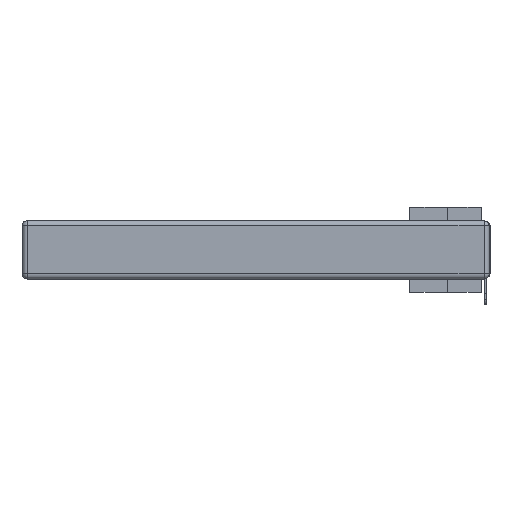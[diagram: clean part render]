
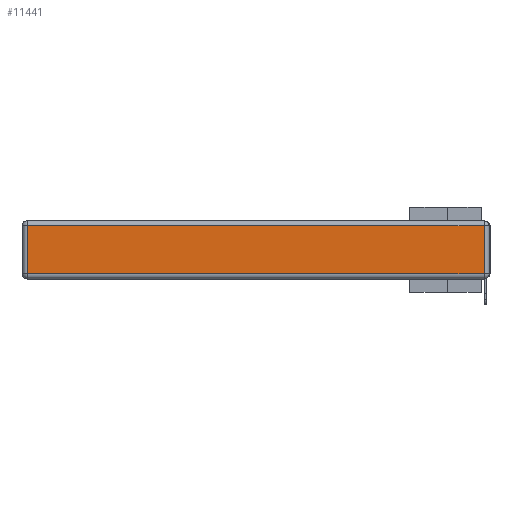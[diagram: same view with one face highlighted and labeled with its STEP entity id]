
A CAD part, left-side view. The second image highlights one B-rep face of the part: STEP entity #11441.
In plain terms, the highlighted planar face has unit normal (-1, 0, 0).
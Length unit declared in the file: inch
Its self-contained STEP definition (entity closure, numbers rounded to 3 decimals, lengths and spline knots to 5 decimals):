
#720 = LINE ( 'NONE', #28766, #16101 ) ;
#1318 = VERTEX_POINT ( 'NONE', #7488 ) ;
#3159 = ORIENTED_EDGE ( 'NONE', *, *, #16158, .T. ) ;
#4341 = DIRECTION ( 'NONE',  ( 0., 0., 1. ) ) ;
#7259 = VECTOR ( 'NONE', #16710, 39.37008 ) ;
#7416 = ORIENTED_EDGE ( 'NONE', *, *, #13104, .T. ) ;
#7488 = CARTESIAN_POINT ( 'NONE',  ( 0., 2.72, -0.313 ) ) ;
#7515 = CARTESIAN_POINT ( 'NONE',  ( 0., 0.03, -0.03 ) ) ;
#7822 = ORIENTED_EDGE ( 'NONE', *, *, #8214, .T. ) ;
#8214 = EDGE_CURVE ( 'NONE', #15928, #32894, #14979, .T. ) ;
#8232 = CARTESIAN_POINT ( 'NONE',  ( 0., 0., -0.343 ) ) ;
#10651 = PLANE ( 'NONE',  #28773 ) ;
#11441 = ADVANCED_FACE ( 'NONE', ( #14709 ), #10651, .T. ) ;
#11745 = CARTESIAN_POINT ( 'NONE',  ( 0., 2.72, -0.343 ) ) ;
#13104 = EDGE_CURVE ( 'NONE', #21676, #15928, #29478, .T. ) ;
#14709 = FACE_OUTER_BOUND ( 'NONE', #34022, .T. ) ;
#14979 = LINE ( 'NONE', #34029, #7259 ) ;
#15928 = VERTEX_POINT ( 'NONE', #7515 ) ;
#15938 = LINE ( 'NONE', #11745, #30003 ) ;
#16101 = VECTOR ( 'NONE', #34733, 39.37008 ) ;
#16158 = EDGE_CURVE ( 'NONE', #1318, #21676, #720, .T. ) ;
#16471 = ORIENTED_EDGE ( 'NONE', *, *, #27239, .T. ) ;
#16710 = DIRECTION ( 'NONE',  ( 0., 1., 0. ) ) ;
#20856 = VECTOR ( 'NONE', #4341, 39.37008 ) ;
#21676 = VERTEX_POINT ( 'NONE', #33018 ) ;
#21695 = CARTESIAN_POINT ( 'NONE',  ( 0., 0.03, -0.343 ) ) ;
#27239 = EDGE_CURVE ( 'NONE', #32894, #1318, #15938, .T. ) ;
#28766 = CARTESIAN_POINT ( 'NONE',  ( 0., 0., -0.313 ) ) ;
#28773 = AXIS2_PLACEMENT_3D ( 'NONE', #8232, #30905, #36727 ) ;
#29478 = LINE ( 'NONE', #21695, #20856 ) ;
#30003 = VECTOR ( 'NONE', #31988, 39.37008 ) ;
#30905 = DIRECTION ( 'NONE',  ( -1., 0., 0. ) ) ;
#31652 = CARTESIAN_POINT ( 'NONE',  ( 0., 2.72, -0.03 ) ) ;
#31988 = DIRECTION ( 'NONE',  ( 0., 0., -1. ) ) ;
#32894 = VERTEX_POINT ( 'NONE', #31652 ) ;
#33018 = CARTESIAN_POINT ( 'NONE',  ( 0., 0.03, -0.313 ) ) ;
#34022 = EDGE_LOOP ( 'NONE', ( #3159, #7416, #7822, #16471 ) ) ;
#34029 = CARTESIAN_POINT ( 'NONE',  ( 0., 2.75, -0.03 ) ) ;
#34733 = DIRECTION ( 'NONE',  ( 0., -1., 0. ) ) ;
#36727 = DIRECTION ( 'NONE',  ( 0., 0., 1. ) ) ;
